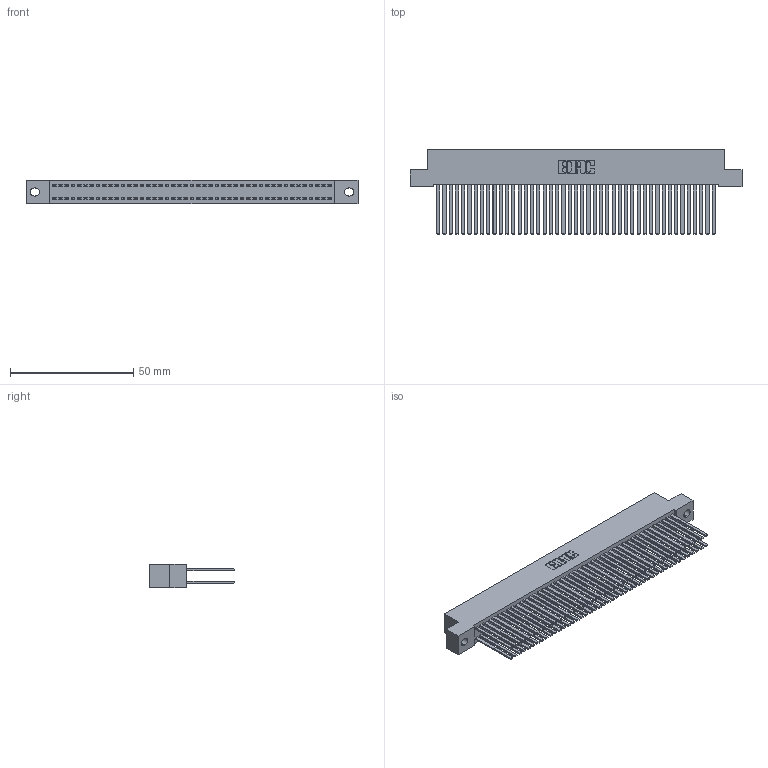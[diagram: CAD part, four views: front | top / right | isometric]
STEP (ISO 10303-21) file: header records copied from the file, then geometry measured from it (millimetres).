
FILE_DESCRIPTION (( 'STEP AP203' ), '1' );
FILE_NAME ('392-090-544-202.STEP', '2018-08-18T07:11:22', ( '' ), ( '' ), 'SwSTEP 2.0', 'SolidWorks 2016', '' );
FILE_SCHEMA (( 'CONFIG_CONTROL_DESIGN' ));
Length unit declared in the file: inch
Products named in the file (3): 345-292-001_345-293-144; 392-090-544-202; 342 Part_.128 Slot
Assembly tree (91 placements, depth 2):
  392-090-544-202
    342 Part_.128 Slot
    345-292-001_345-293-144  x90
Bounding box: 134.62 x 34.3 x 9.4 mm (x, y, z)
Volume: 13319.3 mm3; surface area: 25007.8 mm2
Topology: 91 solids, 91 shells, 4254 faces, 12641 edges, 8306 vertices
Faces by surface type: plane 2950, cylinder 1304
Entity records: 28381 total; most frequent: CARTESIAN_POINT 4698, ORIENTED_EDGE 4634, DIRECTION 4005, EDGE_CURVE 2317, LINE 2193, VECTOR 2193, VERTEX_POINT 1542, AXIS2_PLACEMENT_3D 906
